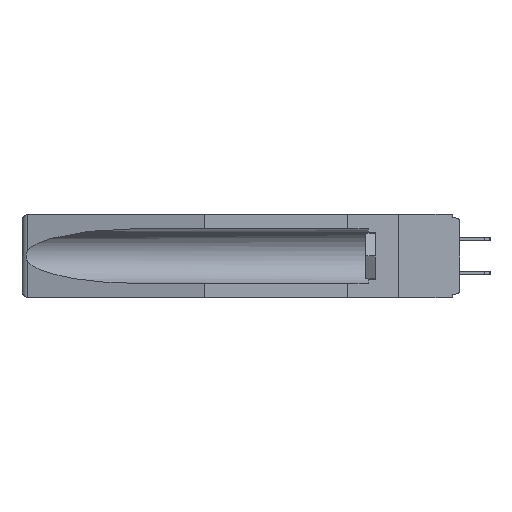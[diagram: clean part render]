
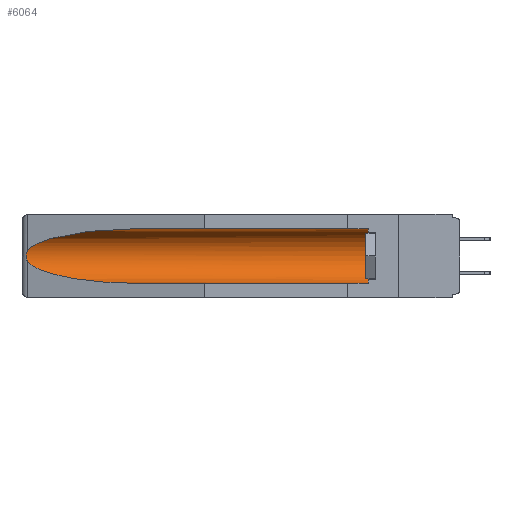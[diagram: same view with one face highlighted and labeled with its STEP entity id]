
A CAD part, left-side view. The second image highlights one B-rep face of the part: STEP entity #6064.
In plain terms, the highlighted cylindrical face has radius 2.857 mm (diameter 5.715 mm), a partial arc.
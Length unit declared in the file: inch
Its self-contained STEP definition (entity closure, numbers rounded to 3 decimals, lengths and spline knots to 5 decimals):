
#933 = CARTESIAN_POINT ( 'NONE',  ( 0.26537, 1.52718, -0.14972 ) ) ;
#1026 = VERTEX_POINT ( 'NONE', #933 ) ;
#1651 = CARTESIAN_POINT ( 'NONE',  ( 0.26537, 1.52718, -0.14972 ) ) ;
#3421 = CARTESIAN_POINT ( 'NONE',  ( 0.155, 0.126, -0.1715 ) ) ;
#3528 = CARTESIAN_POINT ( 'NONE',  ( 0.26537, 1.52718, -0.19328 ) ) ;
#3908 = CARTESIAN_POINT ( 'NONE',  ( 0.25451, 1.48313, -0.09465 ) ) ;
#4345 = CARTESIAN_POINT ( 'NONE',  ( 0.155, 0.126, -0.059 ) ) ;
#4775 = EDGE_LOOP ( 'NONE', ( #11378, #11583, #15271, #23367, #19718, #17269 ) ) ;
#4873 = CARTESIAN_POINT ( 'NONE',  ( 0.155, 1.07973, -0.284 ) ) ;
#5108 = AXIS2_PLACEMENT_3D ( 'NONE', #13506, #15562, #11344 ) ;
#5202 = CARTESIAN_POINT ( 'NONE',  ( 0.26597, 1.52961, -0.15275 ) ) ;
#5789 = DIRECTION ( 'NONE',  ( 0., -1., 0. ) ) ;
#5876 = EDGE_CURVE ( 'NONE', #18815, #25279, #7696, .T. ) ;
#6064 = ADVANCED_FACE ( 'NONE', ( #25003 ), #18720, .F. ) ;
#6171 = CARTESIAN_POINT ( 'NONE',  ( 0.155, 1.07973, -0.059 ) ) ;
#6373 = CARTESIAN_POINT ( 'NONE',  ( 0.26537, 1.52718, -0.19328 ) ) ;
#7296 = CARTESIAN_POINT ( 'NONE',  ( 0.26597, 1.5296, -0.19026 ) ) ;
#7591 = CARTESIAN_POINT ( 'NONE',  ( 0.2675, 1.53308, -0.16763 ) ) ;
#7666 = B_SPLINE_CURVE_WITH_KNOTS ( 'NONE', 3,
 ( #23763, #5202, #21668, #11891, #7591, #24052, #18993, #21358, #7296, #14250 ),
 .UNSPECIFIED., .F., .F.,
 ( 4, 2, 2, 2, 4 ),
 ( 0., 0.00029, 0.00058, 0.00087, 0.00117 ),
 .UNSPECIFIED. ) ;
#7696 = LINE ( 'NONE', #9001, #14645 ) ;
#8590 = VERTEX_POINT ( 'NONE', #11137 ) ;
#8932 = DIRECTION ( 'NONE',  ( 0., 1., 0. ) ) ;
#9001 = CARTESIAN_POINT ( 'NONE',  ( 0.155, -0.30754, -0.059 ) ) ;
#10237 = VECTOR ( 'NONE', #8932, 39.37008 ) ;
#10624 = CARTESIAN_POINT ( 'NONE',  ( 0.25451, 1.48313, -0.24835 ) ) ;
#11095 = CARTESIAN_POINT ( 'NONE',  ( 0.155, 1.07973, -0.059 ) ) ;
#11137 = CARTESIAN_POINT ( 'NONE',  ( 0.155, 0.126, -0.284 ) ) ;
#11344 = DIRECTION ( 'NONE',  ( 0., 0., 1. ) ) ;
#11378 = ORIENTED_EDGE ( 'NONE', *, *, #13389, .T. ) ;
#11583 = ORIENTED_EDGE ( 'NONE', *, *, #30410, .T. ) ;
#11860 = CIRCLE ( 'NONE', #13095, 0.1125 ) ;
#11891 = CARTESIAN_POINT ( 'NONE',  ( 0.2673, 1.5327, -0.16383 ) ) ;
#12293 = VERTEX_POINT ( 'NONE', #6373 ) ;
#13095 = AXIS2_PLACEMENT_3D ( 'NONE', #3421, #5789, #19581 ) ;
#13389 = EDGE_CURVE ( 'NONE', #25279, #1026, #25024, .T. ) ;
#13506 = CARTESIAN_POINT ( 'NONE',  ( 0.155, -0.30754, -0.1715 ) ) ;
#13734 = DIRECTION ( 'NONE',  ( 0., 1., 0. ) ) ;
#14250 = CARTESIAN_POINT ( 'NONE',  ( 0.26537, 1.52718, -0.19328 ) ) ;
#14645 = VECTOR ( 'NONE', #13734, 39.37008 ) ;
#15271 = ORIENTED_EDGE ( 'NONE', *, *, #27504, .T. ) ;
#15562 = DIRECTION ( 'NONE',  ( 0., 1., 0. ) ) ;
#17269 = ORIENTED_EDGE ( 'NONE', *, *, #5876, .T. ) ;
#17988 = CARTESIAN_POINT ( 'NONE',  ( 0.21114, 1.30732, -0.059 ) ) ;
#18183 = CARTESIAN_POINT ( 'NONE',  ( 0.155, -0.30754, -0.284 ) ) ;
#18719 = LINE ( 'NONE', #18183, #10237 ) ;
#18720 = CYLINDRICAL_SURFACE ( 'NONE', #5108, 0.1125 ) ;
#18815 = VERTEX_POINT ( 'NONE', #4345 ) ;
#18993 = CARTESIAN_POINT ( 'NONE',  ( 0.2673, 1.53269, -0.17917 ) ) ;
#19581 = DIRECTION ( 'NONE',  ( 0., 0., 1. ) ) ;
#19718 = ORIENTED_EDGE ( 'NONE', *, *, #25787, .T. ) ;
#20176 = CARTESIAN_POINT ( 'NONE',  ( 0.21114, 1.30732, -0.284 ) ) ;
#21358 = CARTESIAN_POINT ( 'NONE',  ( 0.26655, 1.53094, -0.18657 ) ) ;
#21668 = CARTESIAN_POINT ( 'NONE',  ( 0.26654, 1.53092, -0.15636 ) ) ;
#23363 = VERTEX_POINT ( 'NONE', #4873 ) ;
#23367 = ORIENTED_EDGE ( 'NONE', *, *, #28389, .F. ) ;
#23763 = CARTESIAN_POINT ( 'NONE',  ( 0.26537, 1.52718, -0.14972 ) ) ;
#24052 = CARTESIAN_POINT ( 'NONE',  ( 0.2675, 1.53308, -0.17534 ) ) ;
#24641 =( BOUNDED_CURVE ( )  B_SPLINE_CURVE ( 3, ( #3528, #10624, #20176, #27106 ),
 .UNSPECIFIED., .F., .F. ) 
 B_SPLINE_CURVE_WITH_KNOTS ( ( 4, 4 ),
 ( 0.1948, 1.5708 ),
 .UNSPECIFIED. ) 
 CURVE ( )  GEOMETRIC_REPRESENTATION_ITEM ( )  RATIONAL_B_SPLINE_CURVE ( ( 1., 0.848, 0.848, 1. ) ) 
 REPRESENTATION_ITEM ( '' )  );
#25003 = FACE_OUTER_BOUND ( 'NONE', #4775, .T. ) ;
#25024 =( BOUNDED_CURVE ( )  B_SPLINE_CURVE ( 3, ( #6171, #17988, #3908, #1651 ),
 .UNSPECIFIED., .F., .F. ) 
 B_SPLINE_CURVE_WITH_KNOTS ( ( 4, 4 ),
 ( 4.71239, 6.08839 ),
 .UNSPECIFIED. ) 
 CURVE ( )  GEOMETRIC_REPRESENTATION_ITEM ( )  RATIONAL_B_SPLINE_CURVE ( ( 1., 0.848, 0.848, 1. ) ) 
 REPRESENTATION_ITEM ( '' )  );
#25279 = VERTEX_POINT ( 'NONE', #11095 ) ;
#25787 = EDGE_CURVE ( 'NONE', #8590, #18815, #11860, .T. ) ;
#27106 = CARTESIAN_POINT ( 'NONE',  ( 0.155, 1.07973, -0.284 ) ) ;
#27504 = EDGE_CURVE ( 'NONE', #12293, #23363, #24641, .T. ) ;
#28389 = EDGE_CURVE ( 'NONE', #8590, #23363, #18719, .T. ) ;
#30410 = EDGE_CURVE ( 'NONE', #1026, #12293, #7666, .T. ) ;
